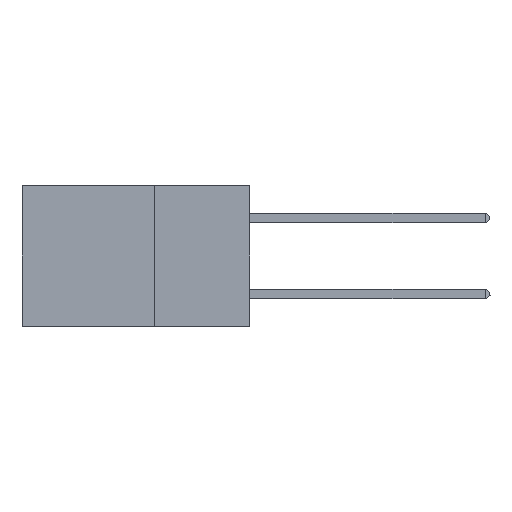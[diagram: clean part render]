
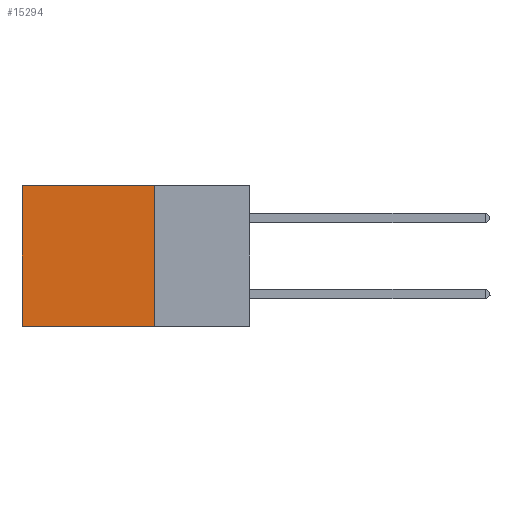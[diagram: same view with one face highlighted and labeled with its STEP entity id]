
A CAD part, left-side view. The second image highlights one B-rep face of the part: STEP entity #15294.
In plain terms, the highlighted planar face has unit normal (-1, 0, 0).
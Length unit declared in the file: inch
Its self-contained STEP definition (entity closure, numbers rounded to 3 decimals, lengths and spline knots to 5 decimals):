
#252 = CARTESIAN_POINT ( 'NONE',  ( 0.2875, 0.25, 0. ) ) ;
#1946 = ORIENTED_EDGE ( 'NONE', *, *, #8884, .F. ) ;
#2353 = CARTESIAN_POINT ( 'NONE',  ( 0.2875, 0.25, 0. ) ) ;
#2859 = VECTOR ( 'NONE', #9704, 39.37008 ) ;
#2870 = VERTEX_POINT ( 'NONE', #13576 ) ;
#3110 = EDGE_CURVE ( 'NONE', #16262, #7829, #13131, .T. ) ;
#3772 = VECTOR ( 'NONE', #9742, 39.37008 ) ;
#4166 = DIRECTION ( 'NONE',  ( 0., 1., 0. ) ) ;
#5041 = EDGE_CURVE ( 'NONE', #2870, #16262, #6247, .T. ) ;
#6014 = DIRECTION ( 'NONE',  ( 0., 0., -1. ) ) ;
#6247 = LINE ( 'NONE', #252, #3772 ) ;
#6335 = VECTOR ( 'NONE', #18616, 39.37008 ) ;
#6446 = CARTESIAN_POINT ( 'NONE',  ( 0.2875, 0.6, 0. ) ) ;
#7829 = VERTEX_POINT ( 'NONE', #10003 ) ;
#8884 = EDGE_CURVE ( 'NONE', #2870, #20127, #12389, .T. ) ;
#9704 = DIRECTION ( 'NONE',  ( 0., 0., -1. ) ) ;
#9742 = DIRECTION ( 'NONE',  ( 0., 1., 0. ) ) ;
#10003 = CARTESIAN_POINT ( 'NONE',  ( 0.2875, 0.6, -0.37 ) ) ;
#11116 = PLANE ( 'NONE',  #19669 ) ;
#11333 = CARTESIAN_POINT ( 'NONE',  ( 0.2875, 0.6, 0. ) ) ;
#11882 = EDGE_LOOP ( 'NONE', ( #18090, #13501, #1946, #16323 ) ) ;
#12389 = LINE ( 'NONE', #18371, #2859 ) ;
#12620 = DIRECTION ( 'NONE',  ( 1., 0., 0. ) ) ;
#13131 = LINE ( 'NONE', #6446, #6335 ) ;
#13501 = ORIENTED_EDGE ( 'NONE', *, *, #18471, .F. ) ;
#13551 = VECTOR ( 'NONE', #4166, 39.37008 ) ;
#13576 = CARTESIAN_POINT ( 'NONE',  ( 0.2875, 0.25, 0. ) ) ;
#13814 = LINE ( 'NONE', #14615, #13551 ) ;
#14615 = CARTESIAN_POINT ( 'NONE',  ( 0.2875, 0.25, -0.37 ) ) ;
#14816 = FACE_OUTER_BOUND ( 'NONE', #11882, .T. ) ;
#15294 = ADVANCED_FACE ( 'NONE', ( #14816 ), #11116, .F. ) ;
#16262 = VERTEX_POINT ( 'NONE', #11333 ) ;
#16323 = ORIENTED_EDGE ( 'NONE', *, *, #5041, .T. ) ;
#18090 = ORIENTED_EDGE ( 'NONE', *, *, #3110, .T. ) ;
#18371 = CARTESIAN_POINT ( 'NONE',  ( 0.2875, 0.25, 0. ) ) ;
#18471 = EDGE_CURVE ( 'NONE', #20127, #7829, #13814, .T. ) ;
#18616 = DIRECTION ( 'NONE',  ( 0., 0., -1. ) ) ;
#19669 = AXIS2_PLACEMENT_3D ( 'NONE', #2353, #12620, #6014 ) ;
#20127 = VERTEX_POINT ( 'NONE', #21263 ) ;
#21263 = CARTESIAN_POINT ( 'NONE',  ( 0.2875, 0.25, -0.37 ) ) ;
